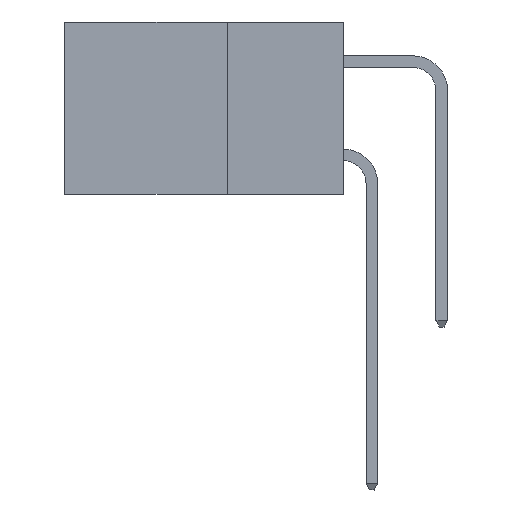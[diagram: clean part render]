
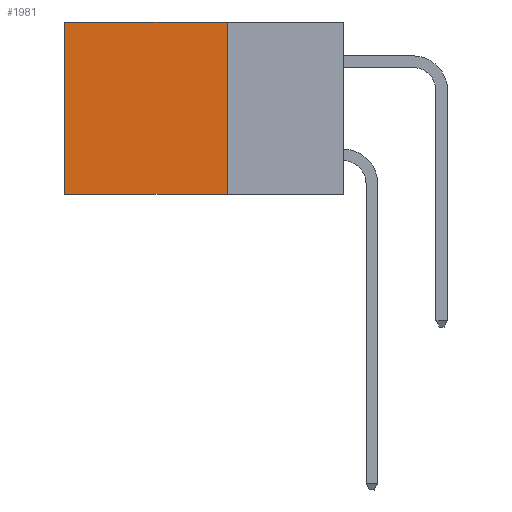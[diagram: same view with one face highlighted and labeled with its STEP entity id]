
A CAD part, left-side view. The second image highlights one B-rep face of the part: STEP entity #1981.
In plain terms, the highlighted planar face has unit normal (-1, 0, 0).
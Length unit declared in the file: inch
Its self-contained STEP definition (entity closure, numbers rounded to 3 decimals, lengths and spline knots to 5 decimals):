
#1806 = VERTEX_POINT ( 'NONE', #6552 ) ;
#1981 = ADVANCED_FACE ( 'NONE', ( #13173 ), #15471, .F. ) ;
#2040 = ORIENTED_EDGE ( 'NONE', *, *, #24892, .T. ) ;
#2183 = CARTESIAN_POINT ( 'NONE',  ( 0.298, 0.25, 0. ) ) ;
#2995 = ORIENTED_EDGE ( 'NONE', *, *, #13359, .F. ) ;
#3151 = DIRECTION ( 'NONE',  ( 0., 1., 0. ) ) ;
#3668 = LINE ( 'NONE', #2183, #11864 ) ;
#4349 = DIRECTION ( 'NONE',  ( 1., 0., 0. ) ) ;
#5484 = DIRECTION ( 'NONE',  ( 0., 0., -1. ) ) ;
#6552 = CARTESIAN_POINT ( 'NONE',  ( 0.298, 0.25, -0.37 ) ) ;
#7136 = DIRECTION ( 'NONE',  ( 0., 0., -1. ) ) ;
#7765 = EDGE_CURVE ( 'NONE', #25199, #24082, #16987, .T. ) ;
#7816 = LINE ( 'NONE', #16356, #17644 ) ;
#8590 = CARTESIAN_POINT ( 'NONE',  ( 0.298, 0.25, 0. ) ) ;
#8819 = DIRECTION ( 'NONE',  ( 0., 1., 0. ) ) ;
#10603 = LINE ( 'NONE', #19670, #32908 ) ;
#10837 = CARTESIAN_POINT ( 'NONE',  ( 0.298, 0.25, 0. ) ) ;
#11864 = VECTOR ( 'NONE', #19183, 39.37008 ) ;
#13173 = FACE_OUTER_BOUND ( 'NONE', #30117, .T. ) ;
#13359 = EDGE_CURVE ( 'NONE', #25199, #1806, #3668, .T. ) ;
#15471 = PLANE ( 'NONE',  #24938 ) ;
#16356 = CARTESIAN_POINT ( 'NONE',  ( 0.298, 0.6, 0. ) ) ;
#16987 = LINE ( 'NONE', #8590, #32855 ) ;
#17644 = VECTOR ( 'NONE', #5484, 39.37008 ) ;
#19183 = DIRECTION ( 'NONE',  ( 0., 0., -1. ) ) ;
#19670 = CARTESIAN_POINT ( 'NONE',  ( 0.298, 0.25, -0.37 ) ) ;
#20882 = ORIENTED_EDGE ( 'NONE', *, *, #7765, .T. ) ;
#22447 = CARTESIAN_POINT ( 'NONE',  ( 0.298, 0.6, -0.37 ) ) ;
#23811 = CARTESIAN_POINT ( 'NONE',  ( 0.298, 0.25, 0. ) ) ;
#24082 = VERTEX_POINT ( 'NONE', #30962 ) ;
#24892 = EDGE_CURVE ( 'NONE', #24082, #30404, #7816, .T. ) ;
#24938 = AXIS2_PLACEMENT_3D ( 'NONE', #23811, #4349, #7136 ) ;
#25199 = VERTEX_POINT ( 'NONE', #10837 ) ;
#30117 = EDGE_LOOP ( 'NONE', ( #2040, #32770, #2995, #20882 ) ) ;
#30404 = VERTEX_POINT ( 'NONE', #22447 ) ;
#30962 = CARTESIAN_POINT ( 'NONE',  ( 0.298, 0.6, 0. ) ) ;
#31488 = EDGE_CURVE ( 'NONE', #1806, #30404, #10603, .T. ) ;
#32770 = ORIENTED_EDGE ( 'NONE', *, *, #31488, .F. ) ;
#32855 = VECTOR ( 'NONE', #3151, 39.37008 ) ;
#32908 = VECTOR ( 'NONE', #8819, 39.37008 ) ;
